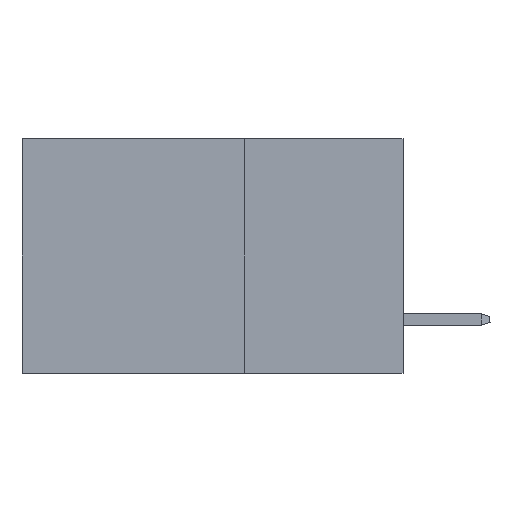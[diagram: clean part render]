
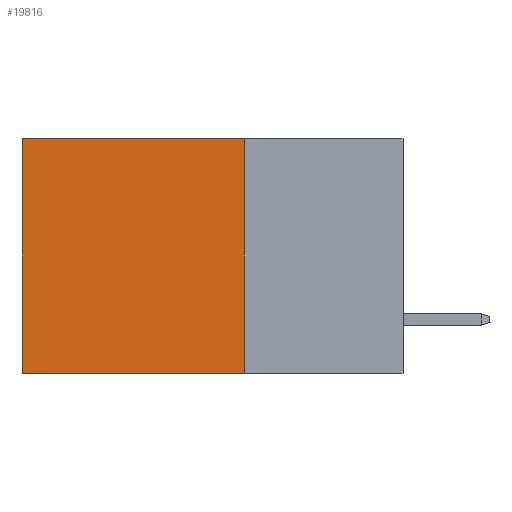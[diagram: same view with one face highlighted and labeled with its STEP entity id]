
A CAD part, left-side view. The second image highlights one B-rep face of the part: STEP entity #19816.
In plain terms, the highlighted planar face has unit normal (-1, 0, 0).
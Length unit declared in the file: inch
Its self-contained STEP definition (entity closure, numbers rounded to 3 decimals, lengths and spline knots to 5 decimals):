
#200 = VERTEX_POINT ( 'NONE', #21067 ) ;
#2647 = ORIENTED_EDGE ( 'NONE', *, *, #18999, .T. ) ;
#3051 = VECTOR ( 'NONE', #20299, 39.37008 ) ;
#3279 = CARTESIAN_POINT ( 'NONE',  ( 0.2875, 0.25, -0.37 ) ) ;
#4429 = VECTOR ( 'NONE', #15358, 39.37008 ) ;
#5431 = VERTEX_POINT ( 'NONE', #12094 ) ;
#6214 = EDGE_LOOP ( 'NONE', ( #10814, #11069, #21915, #2647 ) ) ;
#6543 = CARTESIAN_POINT ( 'NONE',  ( 0.2875, 0.6, 0. ) ) ;
#6654 = PLANE ( 'NONE',  #21431 ) ;
#6767 = DIRECTION ( 'NONE',  ( 1., 0., 0. ) ) ;
#8069 = VECTOR ( 'NONE', #14095, 39.37008 ) ;
#8226 = LINE ( 'NONE', #3279, #4429 ) ;
#9274 = LINE ( 'NONE', #19447, #15127 ) ;
#9690 = CARTESIAN_POINT ( 'NONE',  ( 0.2875, 0.25, -0.37 ) ) ;
#10814 = ORIENTED_EDGE ( 'NONE', *, *, #19915, .T. ) ;
#10853 = DIRECTION ( 'NONE',  ( 0., 0., -1. ) ) ;
#11069 = ORIENTED_EDGE ( 'NONE', *, *, #16087, .F. ) ;
#11880 = EDGE_CURVE ( 'NONE', #14040, #15617, #9274, .T. ) ;
#11938 = CARTESIAN_POINT ( 'NONE',  ( 0.2875, 0.25, 0. ) ) ;
#12094 = CARTESIAN_POINT ( 'NONE',  ( 0.2875, 0.6, 0. ) ) ;
#12614 = CARTESIAN_POINT ( 'NONE',  ( 0.2875, 0.25, 0. ) ) ;
#13412 = FACE_OUTER_BOUND ( 'NONE', #6214, .T. ) ;
#14040 = VERTEX_POINT ( 'NONE', #15170 ) ;
#14095 = DIRECTION ( 'NONE',  ( 0., 1., 0. ) ) ;
#15127 = VECTOR ( 'NONE', #10853, 39.37008 ) ;
#15170 = CARTESIAN_POINT ( 'NONE',  ( 0.2875, 0.25, 0. ) ) ;
#15358 = DIRECTION ( 'NONE',  ( 0., 1., 0. ) ) ;
#15617 = VERTEX_POINT ( 'NONE', #9690 ) ;
#15796 = LINE ( 'NONE', #12614, #8069 ) ;
#16087 = EDGE_CURVE ( 'NONE', #15617, #200, #8226, .T. ) ;
#18999 = EDGE_CURVE ( 'NONE', #14040, #5431, #15796, .T. ) ;
#19447 = CARTESIAN_POINT ( 'NONE',  ( 0.2875, 0.25, 0. ) ) ;
#19816 = ADVANCED_FACE ( 'NONE', ( #13412 ), #6654, .F. ) ;
#19915 = EDGE_CURVE ( 'NONE', #5431, #200, #21720, .T. ) ;
#20299 = DIRECTION ( 'NONE',  ( 0., 0., -1. ) ) ;
#20625 = DIRECTION ( 'NONE',  ( 0., 0., -1. ) ) ;
#21067 = CARTESIAN_POINT ( 'NONE',  ( 0.2875, 0.6, -0.37 ) ) ;
#21431 = AXIS2_PLACEMENT_3D ( 'NONE', #11938, #6767, #20625 ) ;
#21720 = LINE ( 'NONE', #6543, #3051 ) ;
#21915 = ORIENTED_EDGE ( 'NONE', *, *, #11880, .F. ) ;
